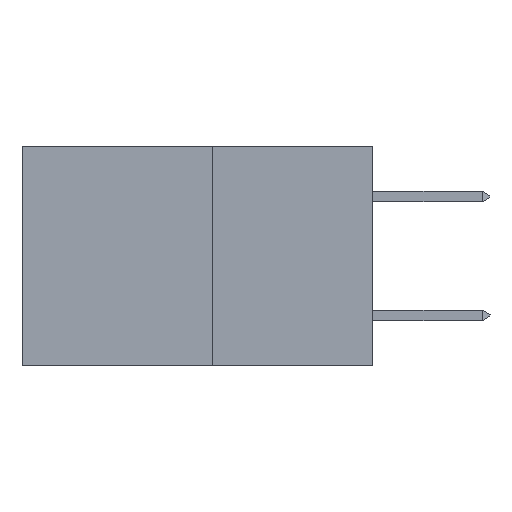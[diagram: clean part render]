
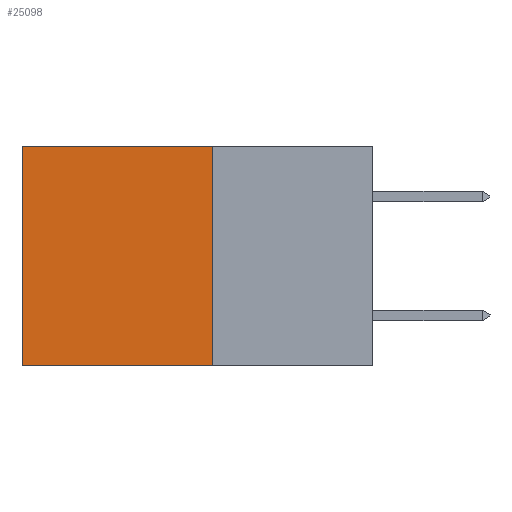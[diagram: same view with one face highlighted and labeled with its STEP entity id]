
A CAD part, left-side view. The second image highlights one B-rep face of the part: STEP entity #25098.
In plain terms, the highlighted planar face has unit normal (-1, 0, 0).
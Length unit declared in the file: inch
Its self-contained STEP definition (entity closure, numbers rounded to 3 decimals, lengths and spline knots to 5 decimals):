
#1253 = DIRECTION ( 'NONE',  ( 0., 1., 0. ) ) ;
#1333 = DIRECTION ( 'NONE',  ( 0., 0., -1. ) ) ;
#1918 = LINE ( 'NONE', #5914, #23161 ) ;
#2543 = AXIS2_PLACEMENT_3D ( 'NONE', #33159, #17301, #1333 ) ;
#4202 = CARTESIAN_POINT ( 'NONE',  ( 0.277, 0.27, -0.37 ) ) ;
#5914 = CARTESIAN_POINT ( 'NONE',  ( 0.277, 0.59, -0.37 ) ) ;
#6687 = VECTOR ( 'NONE', #25469, 39.37008 ) ;
#8600 = DIRECTION ( 'NONE',  ( 0., 0., -1. ) ) ;
#8849 = FACE_OUTER_BOUND ( 'NONE', #26852, .T. ) ;
#9301 = CARTESIAN_POINT ( 'NONE',  ( 0.277, 0.27, 0. ) ) ;
#13021 = CARTESIAN_POINT ( 'NONE',  ( 0.277, 0.27, 0. ) ) ;
#13993 = VERTEX_POINT ( 'NONE', #17603 ) ;
#14675 = EDGE_CURVE ( 'NONE', #24037, #17677, #21943, .T. ) ;
#15283 = VERTEX_POINT ( 'NONE', #17058 ) ;
#15728 = CARTESIAN_POINT ( 'NONE',  ( 0.277, 0.59, 0. ) ) ;
#17058 = CARTESIAN_POINT ( 'NONE',  ( 0.277, 0.27, -0.37 ) ) ;
#17301 = DIRECTION ( 'NONE',  ( 1., 0., 0. ) ) ;
#17603 = CARTESIAN_POINT ( 'NONE',  ( 0.277, 0.59, -0.37 ) ) ;
#17677 = VERTEX_POINT ( 'NONE', #15728 ) ;
#18752 = ORIENTED_EDGE ( 'NONE', *, *, #32982, .F. ) ;
#18991 = VECTOR ( 'NONE', #19823, 39.37008 ) ;
#19823 = DIRECTION ( 'NONE',  ( 0., 1., 0. ) ) ;
#19863 = PLANE ( 'NONE',  #2543 ) ;
#20017 = LINE ( 'NONE', #4202, #6687 ) ;
#20412 = ORIENTED_EDGE ( 'NONE', *, *, #22328, .F. ) ;
#21105 = VECTOR ( 'NONE', #1253, 39.37008 ) ;
#21943 = LINE ( 'NONE', #9301, #21105 ) ;
#22328 = EDGE_CURVE ( 'NONE', #15283, #13993, #33878, .T. ) ;
#23161 = VECTOR ( 'NONE', #8600, 39.37008 ) ;
#24037 = VERTEX_POINT ( 'NONE', #13021 ) ;
#24331 = ORIENTED_EDGE ( 'NONE', *, *, #14675, .T. ) ;
#25098 = ADVANCED_FACE ( 'NONE', ( #8849 ), #19863, .F. ) ;
#25469 = DIRECTION ( 'NONE',  ( 0., 0., -1. ) ) ;
#26852 = EDGE_LOOP ( 'NONE', ( #33441, #20412, #18752, #24331 ) ) ;
#32982 = EDGE_CURVE ( 'NONE', #24037, #15283, #20017, .T. ) ;
#33004 = CARTESIAN_POINT ( 'NONE',  ( 0.277, 0.27, -0.37 ) ) ;
#33159 = CARTESIAN_POINT ( 'NONE',  ( 0.277, 0.27, -0.37 ) ) ;
#33413 = EDGE_CURVE ( 'NONE', #17677, #13993, #1918, .T. ) ;
#33441 = ORIENTED_EDGE ( 'NONE', *, *, #33413, .T. ) ;
#33878 = LINE ( 'NONE', #33004, #18991 ) ;
